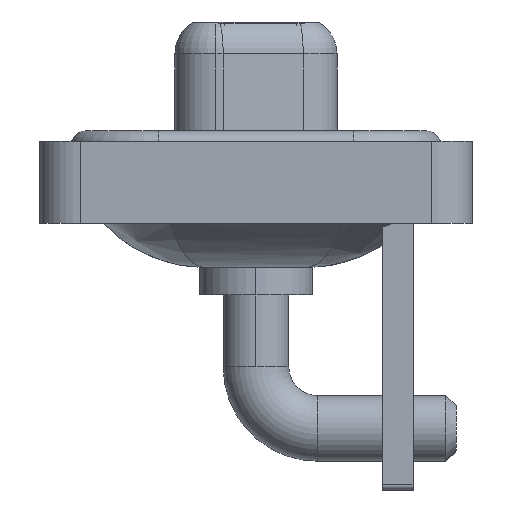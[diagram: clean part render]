
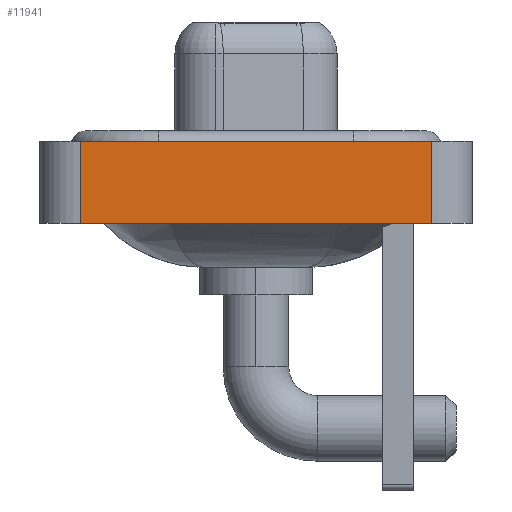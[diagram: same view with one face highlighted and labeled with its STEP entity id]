
A CAD part, left-side view. The second image highlights one B-rep face of the part: STEP entity #11941.
In plain terms, the highlighted planar face has unit normal (-1, 0, 0).
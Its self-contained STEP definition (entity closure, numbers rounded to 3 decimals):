
#245 = CARTESIAN_POINT ( 'NONE',  ( -7.3, -8.55, 0.4 ) ) ;
#361 = CARTESIAN_POINT ( 'NONE',  ( -7.3, 8.55, 0.4 ) ) ;
#643 = DIRECTION ( 'NONE',  ( 0., 0., 1. ) ) ;
#925 = VERTEX_POINT ( 'NONE', #245 ) ;
#1229 = CARTESIAN_POINT ( 'NONE',  ( -7.3, -8.55, -3.6 ) ) ;
#1390 = VERTEX_POINT ( 'NONE', #361 ) ;
#1661 = ORIENTED_EDGE ( 'NONE', *, *, #5199, .F. ) ;
#2381 = LINE ( 'NONE', #6020, #8971 ) ;
#2583 = CARTESIAN_POINT ( 'NONE',  ( -7.3, 8.55, -3.6 ) ) ;
#3347 = CARTESIAN_POINT ( 'NONE',  ( -7.3, -8.55, -3.6 ) ) ;
#3625 = EDGE_CURVE ( 'NONE', #15466, #925, #9041, .T. ) ;
#4209 = PLANE ( 'NONE',  #13755 ) ;
#4530 = CARTESIAN_POINT ( 'NONE',  ( -7.3, -8.55, -3.6 ) ) ;
#5073 = CARTESIAN_POINT ( 'NONE',  ( -7.3, 8.55, -3.6 ) ) ;
#5199 = EDGE_CURVE ( 'NONE', #1390, #925, #2381, .T. ) ;
#5936 = DIRECTION ( 'NONE',  ( 0., -1., 0. ) ) ;
#6020 = CARTESIAN_POINT ( 'NONE',  ( -7.3, -8.55, 0.4 ) ) ;
#6216 = DIRECTION ( 'NONE',  ( 0., 0., 1. ) ) ;
#6361 = VECTOR ( 'NONE', #6216, 1000. ) ;
#6509 = DIRECTION ( 'NONE',  ( 0., 0., 1. ) ) ;
#6576 = CARTESIAN_POINT ( 'NONE',  ( -7.3, -8.55, -3.6 ) ) ;
#6815 = VERTEX_POINT ( 'NONE', #2583 ) ;
#7706 = EDGE_CURVE ( 'NONE', #6815, #15466, #10172, .T. ) ;
#8227 = VECTOR ( 'NONE', #6509, 1000. ) ;
#8678 = ORIENTED_EDGE ( 'NONE', *, *, #7706, .T. ) ;
#8971 = VECTOR ( 'NONE', #5936, 1000. ) ;
#9041 = LINE ( 'NONE', #1229, #6361 ) ;
#9558 = EDGE_CURVE ( 'NONE', #6815, #1390, #14474, .T. ) ;
#9567 = FACE_OUTER_BOUND ( 'NONE', #11368, .T. ) ;
#9966 = ORIENTED_EDGE ( 'NONE', *, *, #9558, .F. ) ;
#10172 = LINE ( 'NONE', #6576, #14713 ) ;
#10211 = ORIENTED_EDGE ( 'NONE', *, *, #3625, .T. ) ;
#11368 = EDGE_LOOP ( 'NONE', ( #10211, #1661, #9966, #8678 ) ) ;
#11941 = ADVANCED_FACE ( 'NONE', ( #9567 ), #4209, .T. ) ;
#13512 = DIRECTION ( 'NONE',  ( -1., 0., 0. ) ) ;
#13755 = AXIS2_PLACEMENT_3D ( 'NONE', #4530, #13512, #643 ) ;
#14191 = DIRECTION ( 'NONE',  ( 0., -1., 0. ) ) ;
#14474 = LINE ( 'NONE', #5073, #8227 ) ;
#14713 = VECTOR ( 'NONE', #14191, 1000. ) ;
#15466 = VERTEX_POINT ( 'NONE', #3347 ) ;
